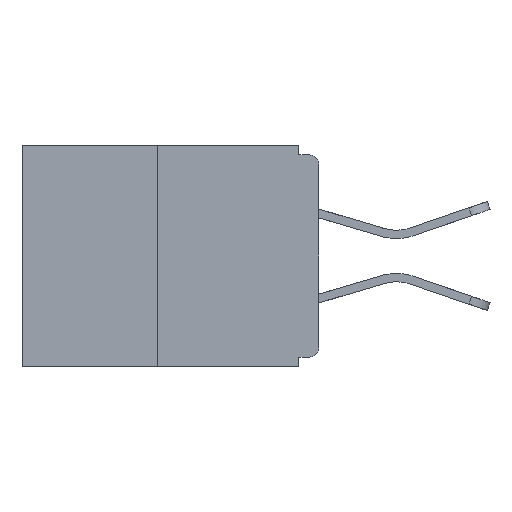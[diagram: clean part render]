
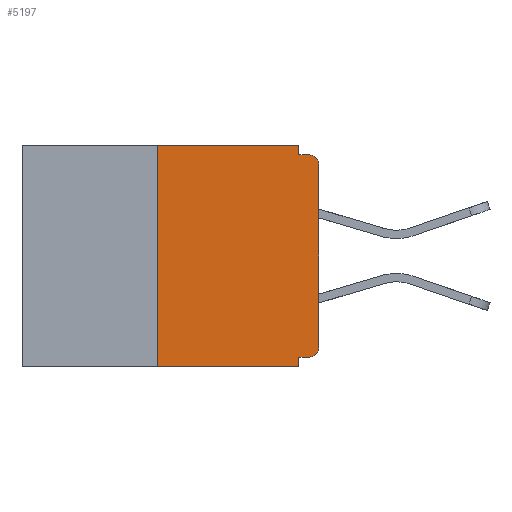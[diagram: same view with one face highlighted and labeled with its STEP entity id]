
A CAD part, left-side view. The second image highlights one B-rep face of the part: STEP entity #5197.
In plain terms, the highlighted planar face has unit normal (-1, 0, 0).
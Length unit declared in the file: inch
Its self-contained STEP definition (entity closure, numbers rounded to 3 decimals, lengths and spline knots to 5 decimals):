
#805 = DIRECTION ( 'NONE',  ( 1., 0., 0. ) ) ;
#1274 = LINE ( 'NONE', #15551, #25513 ) ;
#1600 = CARTESIAN_POINT ( 'NONE',  ( 0., 0., -0.015 ) ) ;
#1816 = CARTESIAN_POINT ( 'NONE',  ( 0., 0.25, 0. ) ) ;
#1952 = ORIENTED_EDGE ( 'NONE', *, *, #21225, .T. ) ;
#2240 = CARTESIAN_POINT ( 'NONE',  ( 0., 0., -0.03 ) ) ;
#2628 = DIRECTION ( 'NONE',  ( 0., 1., 0. ) ) ;
#3012 = VERTEX_POINT ( 'NONE', #14645 ) ;
#3391 = CARTESIAN_POINT ( 'NONE',  ( 0., 0., 0. ) ) ;
#3445 = VECTOR ( 'NONE', #12727, 39.37008 ) ;
#3478 = ORIENTED_EDGE ( 'NONE', *, *, #21713, .F. ) ;
#4141 = LINE ( 'NONE', #16880, #3445 ) ;
#4519 = CARTESIAN_POINT ( 'NONE',  ( 0., 0.015, -0.015 ) ) ;
#4674 = ORIENTED_EDGE ( 'NONE', *, *, #6156, .T. ) ;
#4693 = CIRCLE ( 'NONE', #22924, 0.015 ) ;
#4811 = DIRECTION ( 'NONE',  ( 0., 0., -1. ) ) ;
#5197 = ADVANCED_FACE ( 'NONE', ( #17115 ), #11229, .F. ) ;
#5802 = LINE ( 'NONE', #1600, #15251 ) ;
#5969 = DIRECTION ( 'NONE',  ( 0., -1., 0. ) ) ;
#5998 = CARTESIAN_POINT ( 'NONE',  ( 0., 0.015, -0.03 ) ) ;
#6156 = EDGE_CURVE ( 'NONE', #16888, #14245, #10345, .T. ) ;
#6423 = EDGE_CURVE ( 'NONE', #17906, #17216, #1274, .T. ) ;
#6589 = ORIENTED_EDGE ( 'NONE', *, *, #9058, .F. ) ;
#7397 = VECTOR ( 'NONE', #2628, 39.37008 ) ;
#7823 = CARTESIAN_POINT ( 'NONE',  ( 0., 0.015, -0.328 ) ) ;
#7853 = DIRECTION ( 'NONE',  ( 0., 0., 1. ) ) ;
#8172 = DIRECTION ( 'NONE',  ( 0., 0., -1. ) ) ;
#8423 = CARTESIAN_POINT ( 'NONE',  ( 0., 0.031, -0.343 ) ) ;
#8712 = CARTESIAN_POINT ( 'NONE',  ( 0., 0., -0.328 ) ) ;
#9058 = EDGE_CURVE ( 'NONE', #3012, #27741, #12203, .T. ) ;
#9368 = ORIENTED_EDGE ( 'NONE', *, *, #17816, .T. ) ;
#9511 = EDGE_CURVE ( 'NONE', #24605, #16756, #4141, .T. ) ;
#9531 = ORIENTED_EDGE ( 'NONE', *, *, #11033, .T. ) ;
#10345 = LINE ( 'NONE', #3391, #14693 ) ;
#11033 = EDGE_CURVE ( 'NONE', #16537, #16888, #4693, .T. ) ;
#11229 = PLANE ( 'NONE',  #21094 ) ;
#11447 = VECTOR ( 'NONE', #15661, 39.37008 ) ;
#11905 = CARTESIAN_POINT ( 'NONE',  ( 0., 0.031, 0. ) ) ;
#12014 = CARTESIAN_POINT ( 'NONE',  ( 0., 0.25, 0. ) ) ;
#12106 = DIRECTION ( 'NONE',  ( 0., -1., 0. ) ) ;
#12185 = ORIENTED_EDGE ( 'NONE', *, *, #9511, .F. ) ;
#12203 = LINE ( 'NONE', #1816, #26628 ) ;
#12727 = DIRECTION ( 'NONE',  ( 0., 0., -1. ) ) ;
#13020 = DIRECTION ( 'NONE',  ( 0., 0., -1. ) ) ;
#13175 = LINE ( 'NONE', #25015, #16898 ) ;
#13389 = DIRECTION ( 'NONE',  ( 0., 0., 1. ) ) ;
#13639 = AXIS2_PLACEMENT_3D ( 'NONE', #5998, #23290, #8172 ) ;
#14060 = EDGE_LOOP ( 'NONE', ( #3478, #6589, #1952, #21138, #22790, #9531, #4674, #9368, #22776, #12185 ) ) ;
#14245 = VERTEX_POINT ( 'NONE', #2240 ) ;
#14645 = CARTESIAN_POINT ( 'NONE',  ( 0., 0.25, -0.343 ) ) ;
#14693 = VECTOR ( 'NONE', #13389, 39.37008 ) ;
#15251 = VECTOR ( 'NONE', #12106, 39.37008 ) ;
#15551 = CARTESIAN_POINT ( 'NONE',  ( 0., 0.031, -0.343 ) ) ;
#15661 = DIRECTION ( 'NONE',  ( 0., -1., 0. ) ) ;
#15689 = CARTESIAN_POINT ( 'NONE',  ( 0., 0.031, -0.015 ) ) ;
#16129 = EDGE_CURVE ( 'NONE', #16537, #17906, #18562, .T. ) ;
#16537 = VERTEX_POINT ( 'NONE', #7823 ) ;
#16756 = VERTEX_POINT ( 'NONE', #15689 ) ;
#16880 = CARTESIAN_POINT ( 'NONE',  ( 0., 0.031, 0. ) ) ;
#16888 = VERTEX_POINT ( 'NONE', #26296 ) ;
#16898 = VECTOR ( 'NONE', #5969, 39.37008 ) ;
#17115 = FACE_OUTER_BOUND ( 'NONE', #14060, .T. ) ;
#17212 = LINE ( 'NONE', #20064, #11447 ) ;
#17216 = VERTEX_POINT ( 'NONE', #8423 ) ;
#17267 = CARTESIAN_POINT ( 'NONE',  ( 0., 0.015, -0.313 ) ) ;
#17816 = EDGE_CURVE ( 'NONE', #14245, #18649, #21764, .T. ) ;
#17848 = DIRECTION ( 'NONE',  ( 0., 0., -1. ) ) ;
#17906 = VERTEX_POINT ( 'NONE', #20827 ) ;
#18562 = LINE ( 'NONE', #8712, #7397 ) ;
#18649 = VERTEX_POINT ( 'NONE', #4519 ) ;
#19809 = CARTESIAN_POINT ( 'NONE',  ( 0., 0.46, 0. ) ) ;
#20064 = CARTESIAN_POINT ( 'NONE',  ( 0., 0.46, 0. ) ) ;
#20827 = CARTESIAN_POINT ( 'NONE',  ( 0., 0.031, -0.328 ) ) ;
#21094 = AXIS2_PLACEMENT_3D ( 'NONE', #19809, #805, #17848 ) ;
#21138 = ORIENTED_EDGE ( 'NONE', *, *, #6423, .F. ) ;
#21225 = EDGE_CURVE ( 'NONE', #3012, #17216, #13175, .T. ) ;
#21713 = EDGE_CURVE ( 'NONE', #27741, #24605, #17212, .T. ) ;
#21764 = CIRCLE ( 'NONE', #13639, 0.015 ) ;
#22776 = ORIENTED_EDGE ( 'NONE', *, *, #26428, .F. ) ;
#22790 = ORIENTED_EDGE ( 'NONE', *, *, #16129, .F. ) ;
#22924 = AXIS2_PLACEMENT_3D ( 'NONE', #17267, #25907, #13020 ) ;
#23290 = DIRECTION ( 'NONE',  ( -1., 0., 0. ) ) ;
#24605 = VERTEX_POINT ( 'NONE', #11905 ) ;
#25015 = CARTESIAN_POINT ( 'NONE',  ( 0., 0.46, -0.343 ) ) ;
#25513 = VECTOR ( 'NONE', #4811, 39.37008 ) ;
#25907 = DIRECTION ( 'NONE',  ( -1., 0., 0. ) ) ;
#26296 = CARTESIAN_POINT ( 'NONE',  ( 0., 0., -0.313 ) ) ;
#26428 = EDGE_CURVE ( 'NONE', #16756, #18649, #5802, .T. ) ;
#26628 = VECTOR ( 'NONE', #7853, 39.37008 ) ;
#27741 = VERTEX_POINT ( 'NONE', #12014 ) ;
